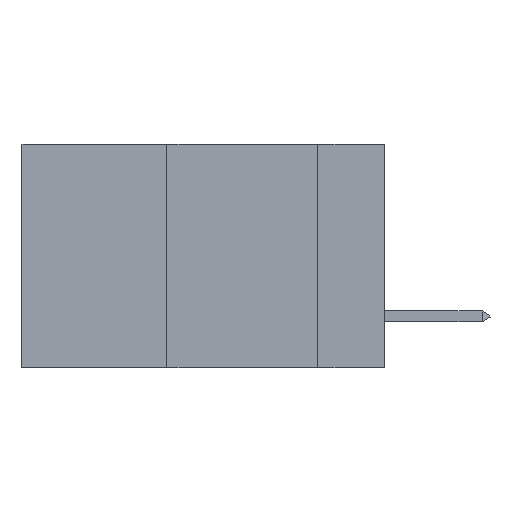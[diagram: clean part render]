
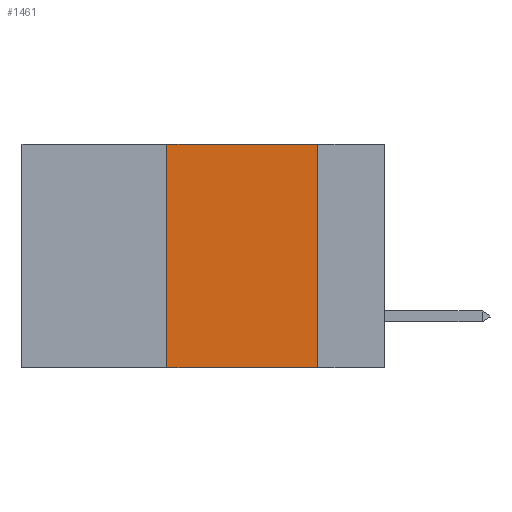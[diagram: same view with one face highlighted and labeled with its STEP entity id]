
A CAD part, left-side view. The second image highlights one B-rep face of the part: STEP entity #1461.
In plain terms, the highlighted planar face has unit normal (-1, 0, 0).
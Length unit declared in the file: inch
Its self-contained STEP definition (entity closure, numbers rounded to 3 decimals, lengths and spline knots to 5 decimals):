
#1073 = CARTESIAN_POINT ( 'NONE',  ( 0., 0.36, 0. ) ) ;
#1273 = LINE ( 'NONE', #6526, #11862 ) ;
#1318 = EDGE_LOOP ( 'NONE', ( #3819, #7385, #10889, #7795 ) ) ;
#1461 = ADVANCED_FACE ( 'NONE', ( #3739 ), #11575, .F. ) ;
#2967 = VERTEX_POINT ( 'NONE', #6982 ) ;
#3259 = DIRECTION ( 'NONE',  ( 1., 0., 0. ) ) ;
#3739 = FACE_OUTER_BOUND ( 'NONE', #1318, .T. ) ;
#3819 = ORIENTED_EDGE ( 'NONE', *, *, #10956, .F. ) ;
#4705 = CARTESIAN_POINT ( 'NONE',  ( 0., 0.6, 0. ) ) ;
#6177 = VECTOR ( 'NONE', #16231, 39.37008 ) ;
#6526 = CARTESIAN_POINT ( 'NONE',  ( 0., 0.6, 0. ) ) ;
#6701 = LINE ( 'NONE', #12941, #16284 ) ;
#6847 = CARTESIAN_POINT ( 'NONE',  ( 0., 0.11, 0. ) ) ;
#6982 = CARTESIAN_POINT ( 'NONE',  ( 0., 0.11, -0.37 ) ) ;
#7385 = ORIENTED_EDGE ( 'NONE', *, *, #12409, .F. ) ;
#7744 = AXIS2_PLACEMENT_3D ( 'NONE', #4705, #3259, #11746 ) ;
#7795 = ORIENTED_EDGE ( 'NONE', *, *, #12972, .T. ) ;
#8339 = VERTEX_POINT ( 'NONE', #15551 ) ;
#8452 = CARTESIAN_POINT ( 'NONE',  ( 0., 0.36, 0. ) ) ;
#9574 = EDGE_CURVE ( 'NONE', #8339, #13008, #13164, .T. ) ;
#10696 = VERTEX_POINT ( 'NONE', #6847 ) ;
#10889 = ORIENTED_EDGE ( 'NONE', *, *, #9574, .F. ) ;
#10913 = VECTOR ( 'NONE', #15128, 39.37008 ) ;
#10956 = EDGE_CURVE ( 'NONE', #10696, #2967, #11319, .T. ) ;
#11319 = LINE ( 'NONE', #12527, #10913 ) ;
#11575 = PLANE ( 'NONE',  #7744 ) ;
#11746 = DIRECTION ( 'NONE',  ( 0., 0., -1. ) ) ;
#11862 = VECTOR ( 'NONE', #14376, 39.37008 ) ;
#12409 = EDGE_CURVE ( 'NONE', #13008, #10696, #1273, .T. ) ;
#12527 = CARTESIAN_POINT ( 'NONE',  ( 0., 0.11, 0. ) ) ;
#12941 = CARTESIAN_POINT ( 'NONE',  ( 0., 0.6, -0.37 ) ) ;
#12972 = EDGE_CURVE ( 'NONE', #8339, #2967, #6701, .T. ) ;
#13008 = VERTEX_POINT ( 'NONE', #1073 ) ;
#13164 = LINE ( 'NONE', #8452, #6177 ) ;
#14252 = DIRECTION ( 'NONE',  ( 0., -1., 0. ) ) ;
#14376 = DIRECTION ( 'NONE',  ( 0., -1., 0. ) ) ;
#15128 = DIRECTION ( 'NONE',  ( 0., 0., -1. ) ) ;
#15551 = CARTESIAN_POINT ( 'NONE',  ( 0., 0.36, -0.37 ) ) ;
#16231 = DIRECTION ( 'NONE',  ( 0., 0., 1. ) ) ;
#16284 = VECTOR ( 'NONE', #14252, 39.37008 ) ;
